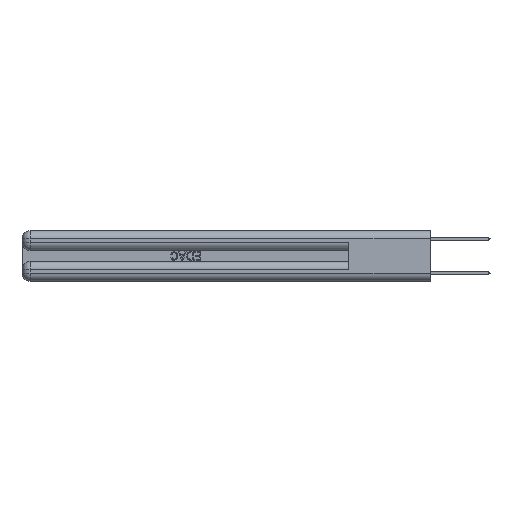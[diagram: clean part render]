
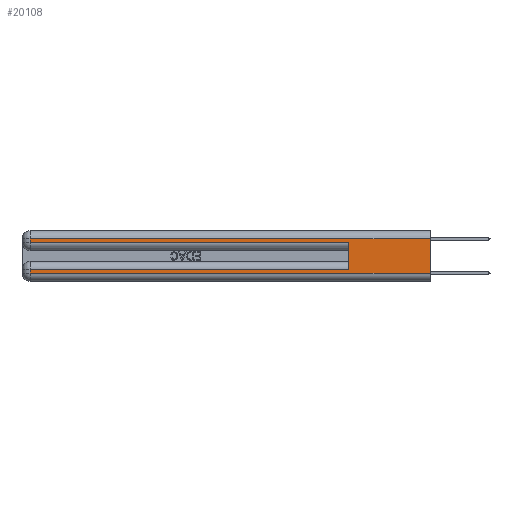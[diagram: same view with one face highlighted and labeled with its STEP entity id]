
A CAD part, left-side view. The second image highlights one B-rep face of the part: STEP entity #20108.
In plain terms, the highlighted planar face has unit normal (-1, 0, 0).
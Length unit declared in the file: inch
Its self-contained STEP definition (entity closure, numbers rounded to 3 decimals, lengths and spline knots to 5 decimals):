
#360 = CARTESIAN_POINT ( 'NONE',  ( 0., 0., 0.06 ) ) ;
#808 = CARTESIAN_POINT ( 'NONE',  ( 0., 2.94, 0.37 ) ) ;
#1155 = VECTOR ( 'NONE', #11643, 39.37008 ) ;
#1311 = DIRECTION ( 'NONE',  ( 0., 1., 0. ) ) ;
#2841 = VERTEX_POINT ( 'NONE', #5074 ) ;
#3860 = ORIENTED_EDGE ( 'NONE', *, *, #17897, .T. ) ;
#4022 = ORIENTED_EDGE ( 'NONE', *, *, #7542, .T. ) ;
#4056 = PLANE ( 'NONE',  #26672 ) ;
#4266 = CARTESIAN_POINT ( 'NONE',  ( 0., 0., 0.285 ) ) ;
#5074 = CARTESIAN_POINT ( 'NONE',  ( 0., 2.94, 0.06 ) ) ;
#5308 = VERTEX_POINT ( 'NONE', #9875 ) ;
#5325 = LINE ( 'NONE', #360, #17649 ) ;
#5866 = LINE ( 'NONE', #25911, #7090 ) ;
#6252 = CARTESIAN_POINT ( 'NONE',  ( 0., 0., 0.37 ) ) ;
#6510 = EDGE_CURVE ( 'NONE', #28580, #2841, #7518, .T. ) ;
#7090 = VECTOR ( 'NONE', #28114, 39.37008 ) ;
#7518 = LINE ( 'NONE', #808, #1155 ) ;
#7542 = EDGE_CURVE ( 'NONE', #20403, #28580, #9807, .T. ) ;
#7746 = CARTESIAN_POINT ( 'NONE',  ( 0., 0., 0.085 ) ) ;
#9644 = ORIENTED_EDGE ( 'NONE', *, *, #24912, .T. ) ;
#9807 = LINE ( 'NONE', #7746, #25077 ) ;
#9875 = CARTESIAN_POINT ( 'NONE',  ( 0., 0., 0.31 ) ) ;
#9971 = ORIENTED_EDGE ( 'NONE', *, *, #15488, .F. ) ;
#10332 = ORIENTED_EDGE ( 'NONE', *, *, #14097, .F. ) ;
#10931 = DIRECTION ( 'NONE',  ( 0., 0., 1. ) ) ;
#11643 = DIRECTION ( 'NONE',  ( 0., 0., -1. ) ) ;
#11987 = CARTESIAN_POINT ( 'NONE',  ( 0., 2.94, 0.285 ) ) ;
#12689 = CARTESIAN_POINT ( 'NONE',  ( 0., 0., 0.37 ) ) ;
#12982 = DIRECTION ( 'NONE',  ( 0., 0., -1. ) ) ;
#13333 = DIRECTION ( 'NONE',  ( 0., -1., 0. ) ) ;
#14055 = CARTESIAN_POINT ( 'NONE',  ( 0., 0., 0.31 ) ) ;
#14097 = EDGE_CURVE ( 'NONE', #5308, #24886, #27923, .T. ) ;
#14538 = ORIENTED_EDGE ( 'NONE', *, *, #23295, .T. ) ;
#15488 = EDGE_CURVE ( 'NONE', #20403, #19395, #22467, .T. ) ;
#15705 = LINE ( 'NONE', #4266, #18559 ) ;
#16050 = EDGE_CURVE ( 'NONE', #2841, #24886, #5325, .T. ) ;
#16259 = LINE ( 'NONE', #14055, #21647 ) ;
#16310 = DIRECTION ( 'NONE',  ( 0., -1., 0. ) ) ;
#17649 = VECTOR ( 'NONE', #16310, 39.37008 ) ;
#17688 = ORIENTED_EDGE ( 'NONE', *, *, #6510, .T. ) ;
#17830 = FACE_OUTER_BOUND ( 'NONE', #25710, .T. ) ;
#17897 = EDGE_CURVE ( 'NONE', #22356, #19395, #15705, .T. ) ;
#18559 = VECTOR ( 'NONE', #13333, 39.37008 ) ;
#18609 = CARTESIAN_POINT ( 'NONE',  ( 0., 0., 0.06 ) ) ;
#19148 = DIRECTION ( 'NONE',  ( 0., 0., -1. ) ) ;
#19395 = VERTEX_POINT ( 'NONE', #23976 ) ;
#20108 = ADVANCED_FACE ( 'NONE', ( #17830 ), #4056, .F. ) ;
#20403 = VERTEX_POINT ( 'NONE', #21428 ) ;
#21098 = CARTESIAN_POINT ( 'NONE',  ( 0., 2.94, 0.31 ) ) ;
#21428 = CARTESIAN_POINT ( 'NONE',  ( 0., 0.6, 0.085 ) ) ;
#21647 = VECTOR ( 'NONE', #27669, 39.37008 ) ;
#22356 = VERTEX_POINT ( 'NONE', #11987 ) ;
#22467 = LINE ( 'NONE', #24383, #23065 ) ;
#23065 = VECTOR ( 'NONE', #10931, 39.37008 ) ;
#23295 = EDGE_CURVE ( 'NONE', #25588, #22356, #5866, .T. ) ;
#23976 = CARTESIAN_POINT ( 'NONE',  ( 0., 0.6, 0.285 ) ) ;
#24383 = CARTESIAN_POINT ( 'NONE',  ( 0., 0.6, 0.145 ) ) ;
#24387 = DIRECTION ( 'NONE',  ( 1., 0., 0. ) ) ;
#24886 = VERTEX_POINT ( 'NONE', #18609 ) ;
#24912 = EDGE_CURVE ( 'NONE', #5308, #25588, #16259, .T. ) ;
#25077 = VECTOR ( 'NONE', #1311, 39.37008 ) ;
#25493 = CARTESIAN_POINT ( 'NONE',  ( 0., 2.94, 0.085 ) ) ;
#25588 = VERTEX_POINT ( 'NONE', #21098 ) ;
#25710 = EDGE_LOOP ( 'NONE', ( #10332, #9644, #14538, #3860, #9971, #4022, #17688, #28139 ) ) ;
#25911 = CARTESIAN_POINT ( 'NONE',  ( 0., 2.94, 0.37 ) ) ;
#26403 = VECTOR ( 'NONE', #19148, 39.37008 ) ;
#26672 = AXIS2_PLACEMENT_3D ( 'NONE', #6252, #24387, #12982 ) ;
#27669 = DIRECTION ( 'NONE',  ( 0., 1., 0. ) ) ;
#27923 = LINE ( 'NONE', #12689, #26403 ) ;
#28114 = DIRECTION ( 'NONE',  ( 0., 0., -1. ) ) ;
#28139 = ORIENTED_EDGE ( 'NONE', *, *, #16050, .T. ) ;
#28580 = VERTEX_POINT ( 'NONE', #25493 ) ;
